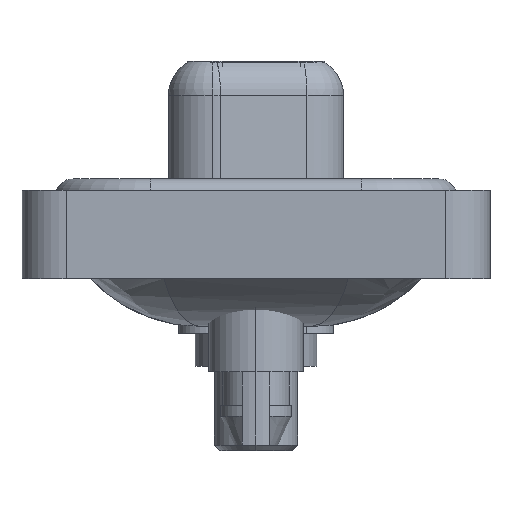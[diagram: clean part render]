
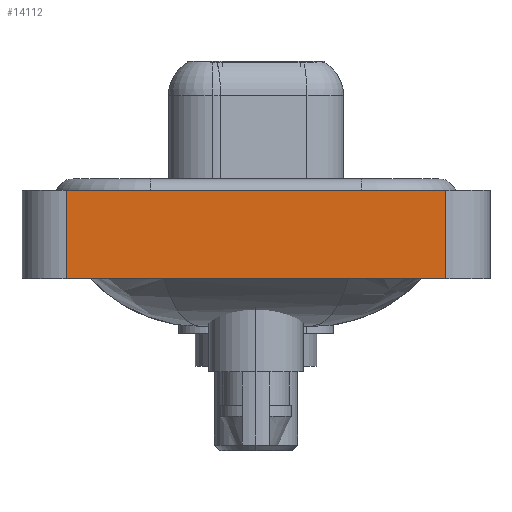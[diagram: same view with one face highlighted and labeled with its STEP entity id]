
A CAD part, left-side view. The second image highlights one B-rep face of the part: STEP entity #14112.
In plain terms, the highlighted planar face has unit normal (-1, 0, 0).
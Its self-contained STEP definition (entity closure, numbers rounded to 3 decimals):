
#136 = CARTESIAN_POINT ( 'NONE',  ( -7.35, -8.55, -3.6 ) ) ;
#764 = VERTEX_POINT ( 'NONE', #3284 ) ;
#989 = LINE ( 'NONE', #6559, #2792 ) ;
#1166 = AXIS2_PLACEMENT_3D ( 'NONE', #9420, #2277, #2370 ) ;
#1403 = ORIENTED_EDGE ( 'NONE', *, *, #11640, .F. ) ;
#2277 = DIRECTION ( 'NONE',  ( -1., 0., 0. ) ) ;
#2370 = DIRECTION ( 'NONE',  ( 0., 0., 1. ) ) ;
#2792 = VECTOR ( 'NONE', #12131, 1000. ) ;
#3284 = CARTESIAN_POINT ( 'NONE',  ( -7.35, 8.55, -3.6 ) ) ;
#3938 = DIRECTION ( 'NONE',  ( 0., -1., 0. ) ) ;
#4618 = EDGE_LOOP ( 'NONE', ( #13452, #16389, #1403, #17786 ) ) ;
#5042 = FACE_OUTER_BOUND ( 'NONE', #4618, .T. ) ;
#5183 = EDGE_CURVE ( 'NONE', #764, #11805, #17914, .T. ) ;
#5895 = LINE ( 'NONE', #11635, #12971 ) ;
#6143 = CARTESIAN_POINT ( 'NONE',  ( -7.35, -8.55, -3.6 ) ) ;
#6559 = CARTESIAN_POINT ( 'NONE',  ( -7.35, -8.55, 0.4 ) ) ;
#8073 = LINE ( 'NONE', #136, #16776 ) ;
#8306 = VERTEX_POINT ( 'NONE', #9282 ) ;
#8972 = DIRECTION ( 'NONE',  ( 0., 0., 1. ) ) ;
#9282 = CARTESIAN_POINT ( 'NONE',  ( -7.35, -8.55, 0.4 ) ) ;
#9420 = CARTESIAN_POINT ( 'NONE',  ( -7.35, -8.55, -3.6 ) ) ;
#9647 = EDGE_CURVE ( 'NONE', #17361, #8306, #989, .T. ) ;
#10591 = EDGE_CURVE ( 'NONE', #11805, #8306, #8073, .T. ) ;
#11635 = CARTESIAN_POINT ( 'NONE',  ( -7.35, 8.55, -3.6 ) ) ;
#11640 = EDGE_CURVE ( 'NONE', #764, #17361, #5895, .T. ) ;
#11805 = VERTEX_POINT ( 'NONE', #6143 ) ;
#12054 = PLANE ( 'NONE',  #1166 ) ;
#12131 = DIRECTION ( 'NONE',  ( 0., -1., 0. ) ) ;
#12620 = DIRECTION ( 'NONE',  ( 0., 0., 1. ) ) ;
#12971 = VECTOR ( 'NONE', #8972, 1000. ) ;
#13452 = ORIENTED_EDGE ( 'NONE', *, *, #10591, .T. ) ;
#13736 = CARTESIAN_POINT ( 'NONE',  ( -7.35, 8.55, 0.4 ) ) ;
#14112 = ADVANCED_FACE ( 'NONE', ( #5042 ), #12054, .T. ) ;
#15704 = VECTOR ( 'NONE', #3938, 1000. ) ;
#16389 = ORIENTED_EDGE ( 'NONE', *, *, #9647, .F. ) ;
#16624 = CARTESIAN_POINT ( 'NONE',  ( -7.35, -8.55, -3.6 ) ) ;
#16776 = VECTOR ( 'NONE', #12620, 1000. ) ;
#17361 = VERTEX_POINT ( 'NONE', #13736 ) ;
#17786 = ORIENTED_EDGE ( 'NONE', *, *, #5183, .T. ) ;
#17914 = LINE ( 'NONE', #16624, #15704 ) ;
